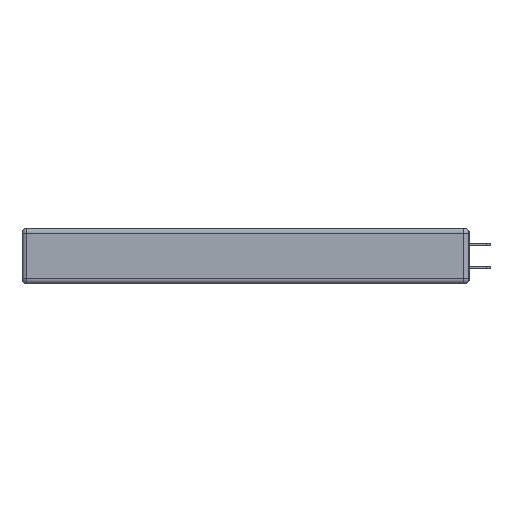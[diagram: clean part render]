
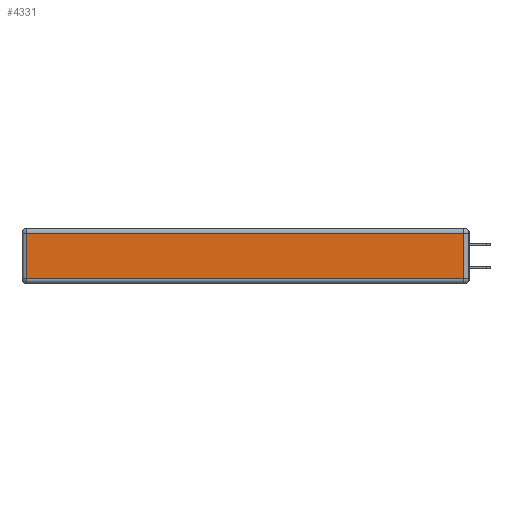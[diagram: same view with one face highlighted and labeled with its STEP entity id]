
A CAD part, left-side view. The second image highlights one B-rep face of the part: STEP entity #4331.
In plain terms, the highlighted planar face has unit normal (-1, 0, 0).
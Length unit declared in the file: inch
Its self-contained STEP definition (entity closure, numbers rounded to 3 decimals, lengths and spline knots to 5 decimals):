
#1626 = CARTESIAN_POINT ( 'NONE',  ( 0., 0.03, -0.343 ) ) ;
#2362 = LINE ( 'NONE', #1626, #17759 ) ;
#3305 = ORIENTED_EDGE ( 'NONE', *, *, #14558, .T. ) ;
#4008 = ORIENTED_EDGE ( 'NONE', *, *, #6337, .T. ) ;
#4190 = ORIENTED_EDGE ( 'NONE', *, *, #18159, .T. ) ;
#4331 = ADVANCED_FACE ( 'NONE', ( #12616 ), #7740, .T. ) ;
#4795 = ORIENTED_EDGE ( 'NONE', *, *, #4889, .T. ) ;
#4889 = EDGE_CURVE ( 'NONE', #16933, #6352, #14701, .T. ) ;
#5086 = DIRECTION ( 'NONE',  ( 0., -1., 0. ) ) ;
#5733 = DIRECTION ( 'NONE',  ( 0., 0., -1. ) ) ;
#5963 = DIRECTION ( 'NONE',  ( 0., 1., 0. ) ) ;
#6141 = CARTESIAN_POINT ( 'NONE',  ( 0., 0.03, -0.03 ) ) ;
#6201 = VERTEX_POINT ( 'NONE', #6141 ) ;
#6337 = EDGE_CURVE ( 'NONE', #13588, #16933, #10692, .T. ) ;
#6352 = VERTEX_POINT ( 'NONE', #18656 ) ;
#7740 = PLANE ( 'NONE',  #13079 ) ;
#8045 = EDGE_LOOP ( 'NONE', ( #4795, #4190, #3305, #4008 ) ) ;
#9222 = CARTESIAN_POINT ( 'NONE',  ( 0., 0., -0.343 ) ) ;
#10561 = DIRECTION ( 'NONE',  ( 0., 0., 1. ) ) ;
#10692 = LINE ( 'NONE', #14681, #14403 ) ;
#10735 = DIRECTION ( 'NONE',  ( -1., 0., 0. ) ) ;
#12214 = DIRECTION ( 'NONE',  ( 0., 0., 1. ) ) ;
#12616 = FACE_OUTER_BOUND ( 'NONE', #8045, .T. ) ;
#12641 = CARTESIAN_POINT ( 'NONE',  ( 0., 2.72, -0.03 ) ) ;
#13079 = AXIS2_PLACEMENT_3D ( 'NONE', #9222, #10735, #12214 ) ;
#13588 = VERTEX_POINT ( 'NONE', #12641 ) ;
#13781 = VECTOR ( 'NONE', #5086, 39.37008 ) ;
#14403 = VECTOR ( 'NONE', #5733, 39.37008 ) ;
#14558 = EDGE_CURVE ( 'NONE', #6201, #13588, #18808, .T. ) ;
#14681 = CARTESIAN_POINT ( 'NONE',  ( 0., 2.72, -0.343 ) ) ;
#14701 = LINE ( 'NONE', #15412, #13781 ) ;
#14836 = VECTOR ( 'NONE', #5963, 39.37008 ) ;
#15412 = CARTESIAN_POINT ( 'NONE',  ( 0., 0., -0.313 ) ) ;
#16445 = CARTESIAN_POINT ( 'NONE',  ( 0., 2.75, -0.03 ) ) ;
#16933 = VERTEX_POINT ( 'NONE', #17615 ) ;
#17615 = CARTESIAN_POINT ( 'NONE',  ( 0., 2.72, -0.313 ) ) ;
#17759 = VECTOR ( 'NONE', #10561, 39.37008 ) ;
#18159 = EDGE_CURVE ( 'NONE', #6352, #6201, #2362, .T. ) ;
#18656 = CARTESIAN_POINT ( 'NONE',  ( 0., 0.03, -0.313 ) ) ;
#18808 = LINE ( 'NONE', #16445, #14836 ) ;
